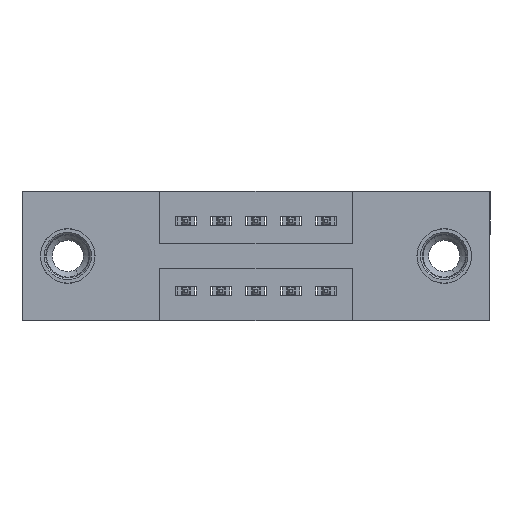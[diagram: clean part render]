
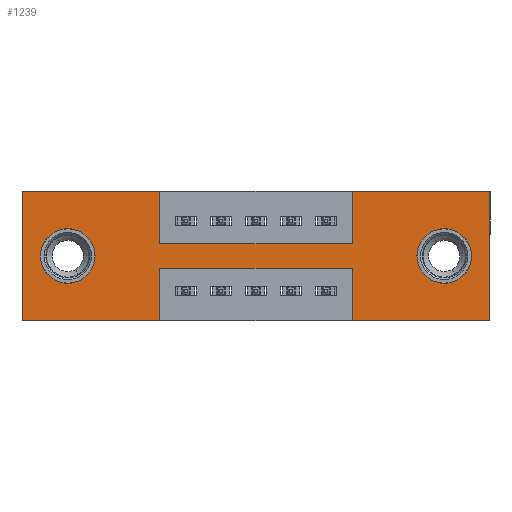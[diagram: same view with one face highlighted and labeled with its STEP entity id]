
A CAD part, front view. The second image highlights one B-rep face of the part: STEP entity #1239.
In plain terms, the highlighted planar face has unit normal (0, -1, 0).
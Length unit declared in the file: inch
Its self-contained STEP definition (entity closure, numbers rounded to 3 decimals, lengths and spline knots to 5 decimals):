
#173 = DIRECTION ( 'NONE',  ( 0., 1., 0. ) ) ;
#216 = ORIENTED_EDGE ( 'NONE', *, *, #10016, .T. ) ;
#367 = ORIENTED_EDGE ( 'NONE', *, *, #12156, .F. ) ;
#371 = EDGE_CURVE ( 'NONE', #3944, #9818, #2770, .T. ) ;
#502 = EDGE_CURVE ( 'NONE', #1086, #9166, #8886, .T. ) ;
#596 = CARTESIAN_POINT ( 'NONE',  ( 1.205, 0., -0.107 ) ) ;
#615 = VERTEX_POINT ( 'NONE', #8377 ) ;
#742 = VERTEX_POINT ( 'NONE', #884 ) ;
#841 = DIRECTION ( 'NONE',  ( 0., 0., -1. ) ) ;
#884 = CARTESIAN_POINT ( 'NONE',  ( 0.3925, 0., -0.15 ) ) ;
#1086 = VERTEX_POINT ( 'NONE', #11359 ) ;
#1239 = ADVANCED_FACE ( 'NONE', ( #10318, #10633, #8250 ), #4011, .T. ) ;
#1280 = CARTESIAN_POINT ( 'NONE',  ( 0.9425, 0., -0.15 ) ) ;
#1352 = VERTEX_POINT ( 'NONE', #13338 ) ;
#1461 = CARTESIAN_POINT ( 'NONE',  ( 1.205, 0., -0.185 ) ) ;
#1500 = DIRECTION ( 'NONE',  ( 0., 1., 0. ) ) ;
#1539 = DIRECTION ( 'NONE',  ( 0., 0., 1. ) ) ;
#1637 = LINE ( 'NONE', #3724, #9772 ) ;
#1853 = VECTOR ( 'NONE', #11188, 39.37008 ) ;
#2048 = EDGE_CURVE ( 'NONE', #9818, #615, #9986, .T. ) ;
#2073 = VECTOR ( 'NONE', #841, 39.37008 ) ;
#2202 = EDGE_LOOP ( 'NONE', ( #7480, #7154, #5670, #8116, #5632, #8577, #11091, #367, #7143, #12361, #4973, #9970 ) ) ;
#2605 = DIRECTION ( 'NONE',  ( 0., 0., -1. ) ) ;
#2668 = LINE ( 'NONE', #9649, #13398 ) ;
#2770 = LINE ( 'NONE', #13331, #2073 ) ;
#2844 = CARTESIAN_POINT ( 'NONE',  ( 0.3925, 0., -0.15 ) ) ;
#2875 = DIRECTION ( 'NONE',  ( 0., 0., -1. ) ) ;
#2894 = CARTESIAN_POINT ( 'NONE',  ( 0., 0., -0.37 ) ) ;
#3192 = EDGE_CURVE ( 'NONE', #9545, #3944, #13510, .T. ) ;
#3347 = DIRECTION ( 'NONE',  ( 0., -1., 0. ) ) ;
#3352 = VERTEX_POINT ( 'NONE', #10032 ) ;
#3371 = CARTESIAN_POINT ( 'NONE',  ( 0.13, 0., -0.185 ) ) ;
#3431 = LINE ( 'NONE', #10580, #11742 ) ;
#3491 = LINE ( 'NONE', #6106, #3839 ) ;
#3608 = ORIENTED_EDGE ( 'NONE', *, *, #502, .T. ) ;
#3688 = DIRECTION ( 'NONE',  ( -1., 0., 0. ) ) ;
#3724 = CARTESIAN_POINT ( 'NONE',  ( 0.3925, 0., 0. ) ) ;
#3826 = LINE ( 'NONE', #2844, #8755 ) ;
#3830 = CARTESIAN_POINT ( 'NONE',  ( 1.335, 0., 0. ) ) ;
#3839 = VECTOR ( 'NONE', #10147, 39.37008 ) ;
#3944 = VERTEX_POINT ( 'NONE', #8641 ) ;
#4011 = PLANE ( 'NONE',  #10846 ) ;
#4118 = LINE ( 'NONE', #13210, #1853 ) ;
#4354 = DIRECTION ( 'NONE',  ( 0., 0., -1. ) ) ;
#4452 = VECTOR ( 'NONE', #5755, 39.37008 ) ;
#4548 = CARTESIAN_POINT ( 'NONE',  ( 0.9425, 0., 0. ) ) ;
#4589 = EDGE_CURVE ( 'NONE', #12776, #1352, #3431, .T. ) ;
#4594 = DIRECTION ( 'NONE',  ( 0., 0., 1. ) ) ;
#4960 = EDGE_CURVE ( 'NONE', #615, #9254, #4118, .T. ) ;
#4973 = ORIENTED_EDGE ( 'NONE', *, *, #4960, .F. ) ;
#5038 = DIRECTION ( 'NONE',  ( 1., 0., 0. ) ) ;
#5384 = LINE ( 'NONE', #9953, #13541 ) ;
#5588 = CIRCLE ( 'NONE', #9630, 0.078 ) ;
#5632 = ORIENTED_EDGE ( 'NONE', *, *, #4589, .F. ) ;
#5670 = ORIENTED_EDGE ( 'NONE', *, *, #10504, .F. ) ;
#5755 = DIRECTION ( 'NONE',  ( -1., 0., 0. ) ) ;
#5825 = CARTESIAN_POINT ( 'NONE',  ( 0.9425, 0., -0.22 ) ) ;
#5986 = DIRECTION ( 'NONE',  ( 0., 1., 0. ) ) ;
#6090 = DIRECTION ( 'NONE',  ( -1., 0., 0. ) ) ;
#6106 = CARTESIAN_POINT ( 'NONE',  ( 0., 0., 0. ) ) ;
#6371 = CARTESIAN_POINT ( 'NONE',  ( 0., 0., 0. ) ) ;
#6572 = LINE ( 'NONE', #13407, #8627 ) ;
#7143 = ORIENTED_EDGE ( 'NONE', *, *, #9603, .F. ) ;
#7154 = ORIENTED_EDGE ( 'NONE', *, *, #3192, .F. ) ;
#7183 = CARTESIAN_POINT ( 'NONE',  ( 0., 0., -0.37 ) ) ;
#7274 = VERTEX_POINT ( 'NONE', #13520 ) ;
#7480 = ORIENTED_EDGE ( 'NONE', *, *, #371, .F. ) ;
#7744 = VERTEX_POINT ( 'NONE', #9398 ) ;
#7968 = CARTESIAN_POINT ( 'NONE',  ( 1.205, 0., -0.185 ) ) ;
#8116 = ORIENTED_EDGE ( 'NONE', *, *, #8965, .F. ) ;
#8122 = CARTESIAN_POINT ( 'NONE',  ( 0., 0., 0. ) ) ;
#8125 = VECTOR ( 'NONE', #6090, 39.37008 ) ;
#8250 = FACE_OUTER_BOUND ( 'NONE', #2202, .T. ) ;
#8270 = ORIENTED_EDGE ( 'NONE', *, *, #8985, .T. ) ;
#8376 = DIRECTION ( 'NONE',  ( 0., 0., 1. ) ) ;
#8377 = CARTESIAN_POINT ( 'NONE',  ( 0., 0., -0.37 ) ) ;
#8577 = ORIENTED_EDGE ( 'NONE', *, *, #11661, .F. ) ;
#8627 = VECTOR ( 'NONE', #8376, 39.37008 ) ;
#8641 = CARTESIAN_POINT ( 'NONE',  ( 0.3925, 0., -0.22 ) ) ;
#8755 = VECTOR ( 'NONE', #5038, 39.37008 ) ;
#8886 = CIRCLE ( 'NONE', #9987, 0.078 ) ;
#8946 = DIRECTION ( 'NONE',  ( 0., 1., 0. ) ) ;
#8950 = VERTEX_POINT ( 'NONE', #4548 ) ;
#8965 = EDGE_CURVE ( 'NONE', #1352, #7744, #5384, .T. ) ;
#8976 = DIRECTION ( 'NONE',  ( 0., 0., -1. ) ) ;
#8985 = EDGE_CURVE ( 'NONE', #3352, #12857, #13214, .T. ) ;
#9089 = VECTOR ( 'NONE', #9129, 39.37008 ) ;
#9120 = AXIS2_PLACEMENT_3D ( 'NONE', #12094, #5986, #13084 ) ;
#9129 = DIRECTION ( 'NONE',  ( 1., 0., 0. ) ) ;
#9166 = VERTEX_POINT ( 'NONE', #9251 ) ;
#9178 = EDGE_LOOP ( 'NONE', ( #216, #8270 ) ) ;
#9232 = EDGE_CURVE ( 'NONE', #12586, #8950, #6572, .T. ) ;
#9251 = CARTESIAN_POINT ( 'NONE',  ( 0.13, 0., -0.107 ) ) ;
#9254 = VERTEX_POINT ( 'NONE', #6371 ) ;
#9398 = CARTESIAN_POINT ( 'NONE',  ( 0.9425, 0., -0.37 ) ) ;
#9543 = ORIENTED_EDGE ( 'NONE', *, *, #10701, .T. ) ;
#9545 = VERTEX_POINT ( 'NONE', #5825 ) ;
#9603 = EDGE_CURVE ( 'NONE', #7274, #742, #1637, .T. ) ;
#9630 = AXIS2_PLACEMENT_3D ( 'NONE', #1461, #8946, #2605 ) ;
#9649 = CARTESIAN_POINT ( 'NONE',  ( 0.9425, 0., -0.37 ) ) ;
#9772 = VECTOR ( 'NONE', #12036, 39.37008 ) ;
#9818 = VERTEX_POINT ( 'NONE', #12385 ) ;
#9914 = CARTESIAN_POINT ( 'NONE',  ( 0.3925, 0., -0.22 ) ) ;
#9953 = CARTESIAN_POINT ( 'NONE',  ( 0., 0., -0.37 ) ) ;
#9970 = ORIENTED_EDGE ( 'NONE', *, *, #2048, .F. ) ;
#9986 = LINE ( 'NONE', #7183, #4452 ) ;
#9987 = AXIS2_PLACEMENT_3D ( 'NONE', #3371, #173, #1539 ) ;
#10016 = EDGE_CURVE ( 'NONE', #12857, #3352, #5588, .T. ) ;
#10032 = CARTESIAN_POINT ( 'NONE',  ( 1.205, 0., -0.263 ) ) ;
#10147 = DIRECTION ( 'NONE',  ( 1., 0., 0. ) ) ;
#10318 = FACE_BOUND ( 'NONE', #9178, .T. ) ;
#10504 = EDGE_CURVE ( 'NONE', #7744, #9545, #2668, .T. ) ;
#10580 = CARTESIAN_POINT ( 'NONE',  ( 1.335, 0., 0. ) ) ;
#10633 = FACE_BOUND ( 'NONE', #11881, .T. ) ;
#10701 = EDGE_CURVE ( 'NONE', #9166, #1086, #11184, .T. ) ;
#10846 = AXIS2_PLACEMENT_3D ( 'NONE', #2894, #3347, #2875 ) ;
#11091 = ORIENTED_EDGE ( 'NONE', *, *, #9232, .F. ) ;
#11184 = CIRCLE ( 'NONE', #9120, 0.078 ) ;
#11188 = DIRECTION ( 'NONE',  ( 0., 0., 1. ) ) ;
#11359 = CARTESIAN_POINT ( 'NONE',  ( 0.13, 0., -0.263 ) ) ;
#11661 = EDGE_CURVE ( 'NONE', #8950, #12776, #12121, .T. ) ;
#11666 = EDGE_CURVE ( 'NONE', #9254, #7274, #3491, .T. ) ;
#11742 = VECTOR ( 'NONE', #4354, 39.37008 ) ;
#11881 = EDGE_LOOP ( 'NONE', ( #9543, #3608 ) ) ;
#12036 = DIRECTION ( 'NONE',  ( 0., 0., -1. ) ) ;
#12094 = CARTESIAN_POINT ( 'NONE',  ( 0.13, 0., -0.185 ) ) ;
#12121 = LINE ( 'NONE', #8122, #9089 ) ;
#12156 = EDGE_CURVE ( 'NONE', #742, #12586, #3826, .T. ) ;
#12361 = ORIENTED_EDGE ( 'NONE', *, *, #11666, .F. ) ;
#12385 = CARTESIAN_POINT ( 'NONE',  ( 0.3925, 0., -0.37 ) ) ;
#12586 = VERTEX_POINT ( 'NONE', #1280 ) ;
#12776 = VERTEX_POINT ( 'NONE', #3830 ) ;
#12857 = VERTEX_POINT ( 'NONE', #596 ) ;
#13084 = DIRECTION ( 'NONE',  ( 0., 0., 1. ) ) ;
#13210 = CARTESIAN_POINT ( 'NONE',  ( 0., 0., 0. ) ) ;
#13214 = CIRCLE ( 'NONE', #13349, 0.078 ) ;
#13331 = CARTESIAN_POINT ( 'NONE',  ( 0.3925, 0., -0.37 ) ) ;
#13338 = CARTESIAN_POINT ( 'NONE',  ( 1.335, 0., -0.37 ) ) ;
#13349 = AXIS2_PLACEMENT_3D ( 'NONE', #7968, #1500, #8976 ) ;
#13398 = VECTOR ( 'NONE', #4594, 39.37008 ) ;
#13407 = CARTESIAN_POINT ( 'NONE',  ( 0.9425, 0., 0. ) ) ;
#13510 = LINE ( 'NONE', #9914, #8125 ) ;
#13520 = CARTESIAN_POINT ( 'NONE',  ( 0.3925, 0., 0. ) ) ;
#13541 = VECTOR ( 'NONE', #3688, 39.37008 ) ;
